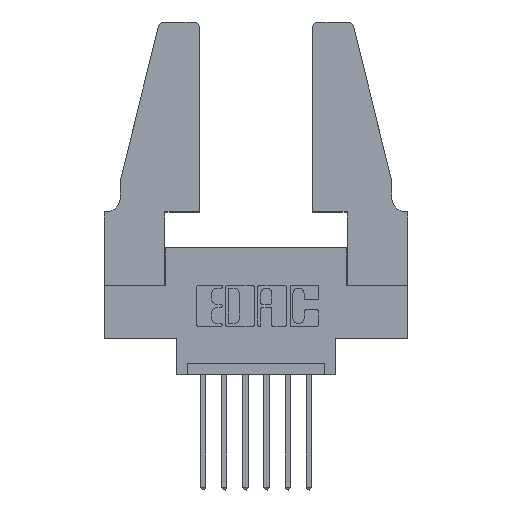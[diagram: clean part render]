
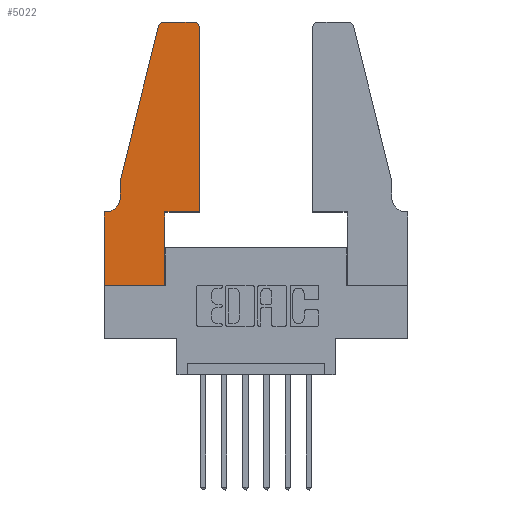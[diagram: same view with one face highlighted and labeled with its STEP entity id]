
A CAD part, top view. The second image highlights one B-rep face of the part: STEP entity #5022.
In plain terms, the highlighted planar face has unit normal (0, 0, 1).
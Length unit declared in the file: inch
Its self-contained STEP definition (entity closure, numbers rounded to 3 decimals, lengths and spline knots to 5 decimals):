
#215 = ORIENTED_EDGE ( 'NONE', *, *, #6647, .T. ) ;
#352 = EDGE_CURVE ( 'NONE', #3309, #4035, #7368, .T. ) ;
#406 = LINE ( 'NONE', #3116, #8022 ) ;
#456 = DIRECTION ( 'NONE',  ( 0., 1., 0. ) ) ;
#618 = CARTESIAN_POINT ( 'NONE',  ( 0., 0.35, 0.37 ) ) ;
#740 = CIRCLE ( 'NONE', #10273, 0.07 ) ;
#822 = EDGE_CURVE ( 'NONE', #5669, #1521, #740, .T. ) ;
#924 = VECTOR ( 'NONE', #4923, 39.37008 ) ;
#1037 = ORIENTED_EDGE ( 'NONE', *, *, #1293, .T. ) ;
#1075 = CARTESIAN_POINT ( 'NONE',  ( 0., 0.35, 0.37 ) ) ;
#1097 = VERTEX_POINT ( 'NONE', #6984 ) ;
#1154 = CARTESIAN_POINT ( 'NONE',  ( 0., 0., 0.37 ) ) ;
#1268 = CARTESIAN_POINT ( 'NONE',  ( 0.0055, 0.35, 0.37 ) ) ;
#1293 = EDGE_CURVE ( 'NONE', #2856, #5231, #3245, .T. ) ;
#1486 = CARTESIAN_POINT ( 'NONE',  ( 0.4505, 0.35, 0.37 ) ) ;
#1521 = VERTEX_POINT ( 'NONE', #1268 ) ;
#1539 = EDGE_CURVE ( 'NONE', #8740, #3974, #406, .T. ) ;
#1656 = CARTESIAN_POINT ( 'NONE',  ( 0.0755, 0.5, 0.37 ) ) ;
#1662 = CIRCLE ( 'NONE', #2153, 0.03 ) ;
#1755 = CARTESIAN_POINT ( 'NONE',  ( 0.0755, 0.5, 0.37 ) ) ;
#2060 = CARTESIAN_POINT ( 'NONE',  ( 0.0755, 0.35, 0.37 ) ) ;
#2153 = AXIS2_PLACEMENT_3D ( 'NONE', #7780, #11341, #8812 ) ;
#2167 = FACE_OUTER_BOUND ( 'NONE', #2721, .T. ) ;
#2256 = CARTESIAN_POINT ( 'NONE',  ( 0.4205, 1.22, 0.37 ) ) ;
#2481 = ORIENTED_EDGE ( 'NONE', *, *, #1539, .T. ) ;
#2646 = ORIENTED_EDGE ( 'NONE', *, *, #9520, .T. ) ;
#2684 = DIRECTION ( 'NONE',  ( 0., -1., 0. ) ) ;
#2721 = EDGE_LOOP ( 'NONE', ( #7158, #8568, #9281, #6776, #10437, #4965, #1037, #2646, #2481, #2735, #9259, #215 ) ) ;
#2735 = ORIENTED_EDGE ( 'NONE', *, *, #5850, .T. ) ;
#2856 = VERTEX_POINT ( 'NONE', #1075 ) ;
#3116 = CARTESIAN_POINT ( 'NONE',  ( 0.2865, 0.35, 0.37 ) ) ;
#3163 = DIRECTION ( 'NONE',  ( 0., 0., 1. ) ) ;
#3236 = DIRECTION ( 'NONE',  ( 1., 0., 0. ) ) ;
#3245 = LINE ( 'NONE', #1154, #10166 ) ;
#3309 = VERTEX_POINT ( 'NONE', #4403 ) ;
#3652 = DIRECTION ( 'NONE',  ( 1., 0., 0. ) ) ;
#3782 = VECTOR ( 'NONE', #4303, 39.37008 ) ;
#3913 = AXIS2_PLACEMENT_3D ( 'NONE', #2256, #3163, #3236 ) ;
#3974 = VERTEX_POINT ( 'NONE', #10345 ) ;
#4035 = VERTEX_POINT ( 'NONE', #5319 ) ;
#4038 = VECTOR ( 'NONE', #2684, 39.37008 ) ;
#4303 = DIRECTION ( 'NONE',  ( 0., 1., 0. ) ) ;
#4345 = LINE ( 'NONE', #1486, #3782 ) ;
#4403 = CARTESIAN_POINT ( 'NONE',  ( 0.25487, 1.22718, 0.37 ) ) ;
#4510 = AXIS2_PLACEMENT_3D ( 'NONE', #618, #6921, #7857 ) ;
#4694 = LINE ( 'NONE', #9015, #6763 ) ;
#4808 = EDGE_CURVE ( 'NONE', #10922, #10782, #11336, .T. ) ;
#4923 = DIRECTION ( 'NONE',  ( -1., 0., 0. ) ) ;
#4963 = CARTESIAN_POINT ( 'NONE',  ( 0., 0., 0.37 ) ) ;
#4965 = ORIENTED_EDGE ( 'NONE', *, *, #7632, .T. ) ;
#5022 = ADVANCED_FACE ( 'NONE', ( #2167 ), #5199, .T. ) ;
#5199 = PLANE ( 'NONE',  #4510 ) ;
#5231 = VERTEX_POINT ( 'NONE', #4963 ) ;
#5319 = CARTESIAN_POINT ( 'NONE',  ( 0.0755, 0.5, 0.37 ) ) ;
#5325 = CARTESIAN_POINT ( 'NONE',  ( 0.284, 1.25, 0.37 ) ) ;
#5327 = VECTOR ( 'NONE', #11478, 39.37008 ) ;
#5468 = CARTESIAN_POINT ( 'NONE',  ( 0.4505, 1.22, 0.37 ) ) ;
#5669 = VERTEX_POINT ( 'NONE', #6192 ) ;
#5709 = EDGE_CURVE ( 'NONE', #4035, #5669, #9684, .T. ) ;
#5719 = VECTOR ( 'NONE', #7467, 39.37008 ) ;
#5804 = EDGE_CURVE ( 'NONE', #10782, #3309, #1662, .T. ) ;
#5850 = EDGE_CURVE ( 'NONE', #3974, #1097, #10112, .T. ) ;
#5943 = EDGE_CURVE ( 'NONE', #1097, #6378, #4345, .T. ) ;
#6192 = CARTESIAN_POINT ( 'NONE',  ( 0.0755, 0.42, 0.37 ) ) ;
#6378 = VERTEX_POINT ( 'NONE', #5468 ) ;
#6647 = EDGE_CURVE ( 'NONE', #6378, #10922, #8829, .T. ) ;
#6763 = VECTOR ( 'NONE', #3652, 39.37008 ) ;
#6776 = ORIENTED_EDGE ( 'NONE', *, *, #5709, .T. ) ;
#6786 = CARTESIAN_POINT ( 'NONE',  ( 0.0055, 0.42, 0.37 ) ) ;
#6921 = DIRECTION ( 'NONE',  ( 0., 0., 1. ) ) ;
#6984 = CARTESIAN_POINT ( 'NONE',  ( 0.4505, 0.35, 0.37 ) ) ;
#7158 = ORIENTED_EDGE ( 'NONE', *, *, #4808, .T. ) ;
#7368 = LINE ( 'NONE', #1656, #9912 ) ;
#7446 = DIRECTION ( 'NONE',  ( 0., -1., 0. ) ) ;
#7467 = DIRECTION ( 'NONE',  ( -1., 0., 0. ) ) ;
#7632 = EDGE_CURVE ( 'NONE', #1521, #2856, #8641, .T. ) ;
#7678 = DIRECTION ( 'NONE',  ( 0., 0., -1. ) ) ;
#7780 = CARTESIAN_POINT ( 'NONE',  ( 0.284, 1.22, 0.37 ) ) ;
#7857 = DIRECTION ( 'NONE',  ( 1., 0., 0. ) ) ;
#8022 = VECTOR ( 'NONE', #456, 39.37008 ) ;
#8037 = CARTESIAN_POINT ( 'NONE',  ( 0.2865, 0., 0.37 ) ) ;
#8568 = ORIENTED_EDGE ( 'NONE', *, *, #5804, .T. ) ;
#8582 = DIRECTION ( 'NONE',  ( -1., 0., 0. ) ) ;
#8641 = LINE ( 'NONE', #2060, #5719 ) ;
#8740 = VERTEX_POINT ( 'NONE', #8037 ) ;
#8812 = DIRECTION ( 'NONE',  ( 1., 0., 0. ) ) ;
#8829 = CIRCLE ( 'NONE', #3913, 0.03 ) ;
#9015 = CARTESIAN_POINT ( 'NONE',  ( 0., 0., 0.37 ) ) ;
#9245 = CARTESIAN_POINT ( 'NONE',  ( 0.2605, 1.25, 0.37 ) ) ;
#9259 = ORIENTED_EDGE ( 'NONE', *, *, #5943, .T. ) ;
#9281 = ORIENTED_EDGE ( 'NONE', *, *, #352, .T. ) ;
#9520 = EDGE_CURVE ( 'NONE', #5231, #8740, #4694, .T. ) ;
#9684 = LINE ( 'NONE', #1755, #4038 ) ;
#9801 = DIRECTION ( 'NONE',  ( -0.239, -0.971, 0. ) ) ;
#9912 = VECTOR ( 'NONE', #9801, 39.37008 ) ;
#10112 = LINE ( 'NONE', #10567, #5327 ) ;
#10122 = CARTESIAN_POINT ( 'NONE',  ( 0.4205, 1.25, 0.37 ) ) ;
#10166 = VECTOR ( 'NONE', #7446, 39.37008 ) ;
#10273 = AXIS2_PLACEMENT_3D ( 'NONE', #6786, #7678, #8582 ) ;
#10345 = CARTESIAN_POINT ( 'NONE',  ( 0.2865, 0.35, 0.37 ) ) ;
#10437 = ORIENTED_EDGE ( 'NONE', *, *, #822, .T. ) ;
#10567 = CARTESIAN_POINT ( 'NONE',  ( 0.4505, 0.35, 0.37 ) ) ;
#10782 = VERTEX_POINT ( 'NONE', #5325 ) ;
#10922 = VERTEX_POINT ( 'NONE', #10122 ) ;
#11336 = LINE ( 'NONE', #9245, #924 ) ;
#11341 = DIRECTION ( 'NONE',  ( 0., 0., 1. ) ) ;
#11478 = DIRECTION ( 'NONE',  ( 1., 0., 0. ) ) ;
